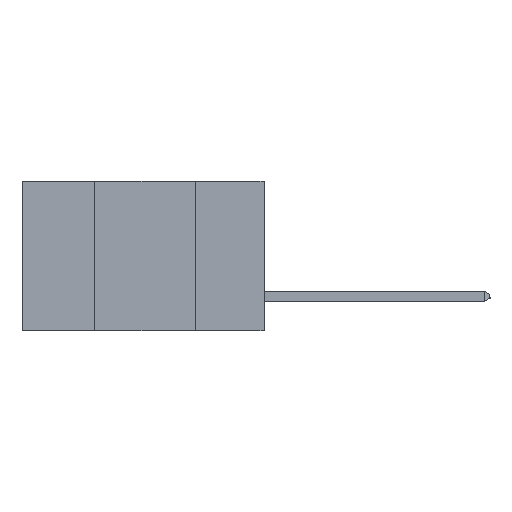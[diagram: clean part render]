
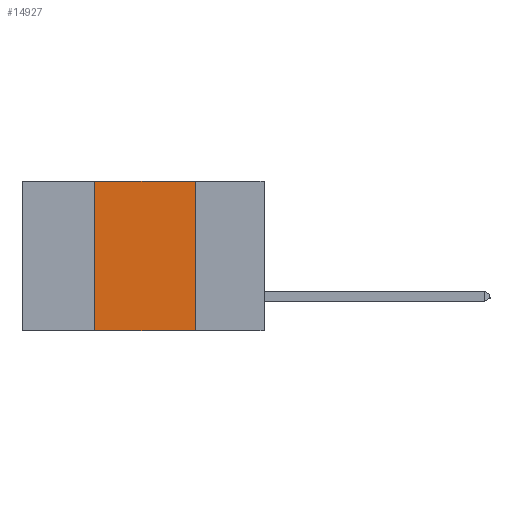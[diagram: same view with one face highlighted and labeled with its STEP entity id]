
A CAD part, left-side view. The second image highlights one B-rep face of the part: STEP entity #14927.
In plain terms, the highlighted planar face has unit normal (-1, 0, 0).
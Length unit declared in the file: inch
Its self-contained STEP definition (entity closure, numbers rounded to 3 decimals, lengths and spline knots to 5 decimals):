
#1742 = VECTOR ( 'NONE', #3407, 39.37008 ) ;
#1751 = CARTESIAN_POINT ( 'NONE',  ( 0., 0.6, -0.37 ) ) ;
#2263 = CARTESIAN_POINT ( 'NONE',  ( 0., 0.6, 0. ) ) ;
#2365 = FACE_OUTER_BOUND ( 'NONE', #21679, .T. ) ;
#3407 = DIRECTION ( 'NONE',  ( 0., -1., 0. ) ) ;
#3997 = LINE ( 'NONE', #25759, #16698 ) ;
#4200 = VERTEX_POINT ( 'NONE', #6982 ) ;
#4879 = EDGE_CURVE ( 'NONE', #11322, #4200, #24940, .T. ) ;
#5519 = ORIENTED_EDGE ( 'NONE', *, *, #9372, .T. ) ;
#6263 = VERTEX_POINT ( 'NONE', #10308 ) ;
#6513 = DIRECTION ( 'NONE',  ( 0., -1., 0. ) ) ;
#6982 = CARTESIAN_POINT ( 'NONE',  ( 0., 0.17, -0.37 ) ) ;
#8145 = ORIENTED_EDGE ( 'NONE', *, *, #4879, .F. ) ;
#9372 = EDGE_CURVE ( 'NONE', #25166, #4200, #30397, .T. ) ;
#10134 = CARTESIAN_POINT ( 'NONE',  ( 0., 0.17, 0. ) ) ;
#10308 = CARTESIAN_POINT ( 'NONE',  ( 0., 0.42, 0. ) ) ;
#10433 = EDGE_CURVE ( 'NONE', #25166, #6263, #3997, .T. ) ;
#11322 = VERTEX_POINT ( 'NONE', #10134 ) ;
#11515 = DIRECTION ( 'NONE',  ( 0., 0., 1. ) ) ;
#13679 = LINE ( 'NONE', #17686, #1742 ) ;
#14255 = DIRECTION ( 'NONE',  ( 1., 0., 0. ) ) ;
#14846 = CARTESIAN_POINT ( 'NONE',  ( 0., 0.17, 0. ) ) ;
#14927 = ADVANCED_FACE ( 'NONE', ( #2365 ), #28431, .F. ) ;
#16000 = ORIENTED_EDGE ( 'NONE', *, *, #18528, .F. ) ;
#16698 = VECTOR ( 'NONE', #11515, 39.37008 ) ;
#17686 = CARTESIAN_POINT ( 'NONE',  ( 0., 0.6, 0. ) ) ;
#17844 = VECTOR ( 'NONE', #6513, 39.37008 ) ;
#18528 = EDGE_CURVE ( 'NONE', #6263, #11322, #13679, .T. ) ;
#19629 = AXIS2_PLACEMENT_3D ( 'NONE', #2263, #14255, #26053 ) ;
#21679 = EDGE_LOOP ( 'NONE', ( #8145, #16000, #23849, #5519 ) ) ;
#23435 = DIRECTION ( 'NONE',  ( 0., 0., -1. ) ) ;
#23849 = ORIENTED_EDGE ( 'NONE', *, *, #10433, .F. ) ;
#24940 = LINE ( 'NONE', #14846, #30419 ) ;
#25038 = CARTESIAN_POINT ( 'NONE',  ( 0., 0.42, -0.37 ) ) ;
#25166 = VERTEX_POINT ( 'NONE', #25038 ) ;
#25759 = CARTESIAN_POINT ( 'NONE',  ( 0., 0.42, 0. ) ) ;
#26053 = DIRECTION ( 'NONE',  ( 0., 0., -1. ) ) ;
#28431 = PLANE ( 'NONE',  #19629 ) ;
#30397 = LINE ( 'NONE', #1751, #17844 ) ;
#30419 = VECTOR ( 'NONE', #23435, 39.37008 ) ;
